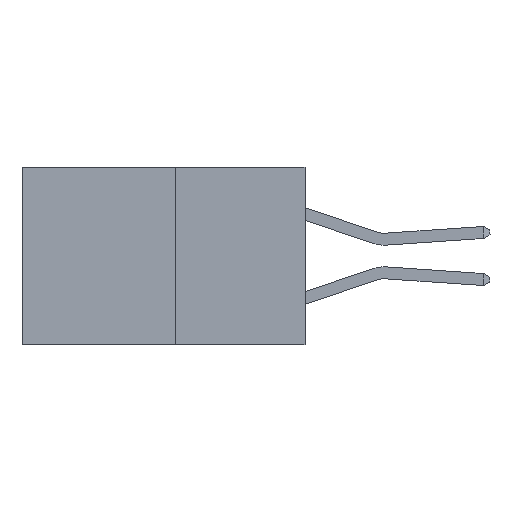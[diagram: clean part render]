
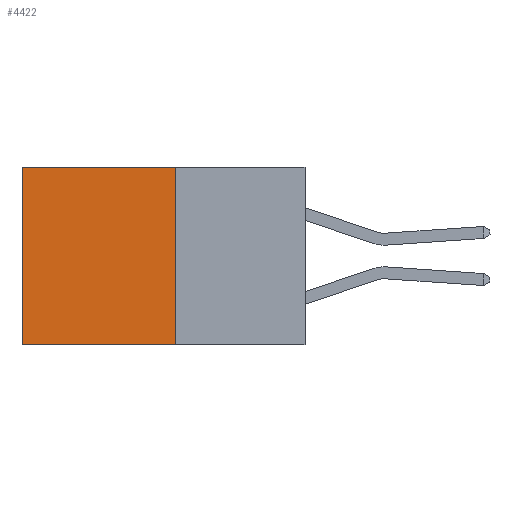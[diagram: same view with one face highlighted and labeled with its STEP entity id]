
A CAD part, left-side view. The second image highlights one B-rep face of the part: STEP entity #4422.
In plain terms, the highlighted planar face has unit normal (-1, 0, 0).
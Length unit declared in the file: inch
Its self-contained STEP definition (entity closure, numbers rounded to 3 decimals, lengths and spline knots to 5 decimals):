
#816 = EDGE_CURVE ( 'NONE', #3870, #5672, #6788, .T. ) ;
#1032 = EDGE_CURVE ( 'NONE', #5672, #4054, #9245, .T. ) ;
#1395 = CARTESIAN_POINT ( 'NONE',  ( 0.277, 0.27, -0.37 ) ) ;
#1865 = CARTESIAN_POINT ( 'NONE',  ( 0.277, 0.59, -0.37 ) ) ;
#2240 = CARTESIAN_POINT ( 'NONE',  ( 0.277, 0.59, 0. ) ) ;
#2380 = CARTESIAN_POINT ( 'NONE',  ( 0.277, 0.27, -0.37 ) ) ;
#2745 = LINE ( 'NONE', #2380, #8759 ) ;
#3063 = EDGE_CURVE ( 'NONE', #7665, #4054, #6095, .T. ) ;
#3579 = CARTESIAN_POINT ( 'NONE',  ( 0.277, 0.59, -0.37 ) ) ;
#3745 = AXIS2_PLACEMENT_3D ( 'NONE', #7727, #7685, #7627 ) ;
#3870 = VERTEX_POINT ( 'NONE', #9996 ) ;
#4031 = FACE_OUTER_BOUND ( 'NONE', #9050, .T. ) ;
#4054 = VERTEX_POINT ( 'NONE', #3579 ) ;
#4422 = ADVANCED_FACE ( 'NONE', ( #4031 ), #7743, .F. ) ;
#4441 = ORIENTED_EDGE ( 'NONE', *, *, #1032, .T. ) ;
#4519 = ORIENTED_EDGE ( 'NONE', *, *, #3063, .F. ) ;
#4556 = ORIENTED_EDGE ( 'NONE', *, *, #5852, .F. ) ;
#4741 = DIRECTION ( 'NONE',  ( 0., 0., -1. ) ) ;
#4990 = CARTESIAN_POINT ( 'NONE',  ( 0.277, 0.27, 0. ) ) ;
#5043 = ORIENTED_EDGE ( 'NONE', *, *, #816, .T. ) ;
#5672 = VERTEX_POINT ( 'NONE', #2240 ) ;
#5852 = EDGE_CURVE ( 'NONE', #3870, #7665, #2745, .T. ) ;
#5855 = VECTOR ( 'NONE', #9581, 39.37008 ) ;
#6095 = LINE ( 'NONE', #1395, #5855 ) ;
#6309 = CARTESIAN_POINT ( 'NONE',  ( 0.277, 0.27, -0.37 ) ) ;
#6533 = VECTOR ( 'NONE', #6803, 39.37008 ) ;
#6788 = LINE ( 'NONE', #4990, #6533 ) ;
#6803 = DIRECTION ( 'NONE',  ( 0., 1., 0. ) ) ;
#7219 = DIRECTION ( 'NONE',  ( 0., 0., -1. ) ) ;
#7627 = DIRECTION ( 'NONE',  ( 0., 0., -1. ) ) ;
#7665 = VERTEX_POINT ( 'NONE', #6309 ) ;
#7685 = DIRECTION ( 'NONE',  ( 1., 0., 0. ) ) ;
#7727 = CARTESIAN_POINT ( 'NONE',  ( 0.277, 0.27, -0.37 ) ) ;
#7743 = PLANE ( 'NONE',  #3745 ) ;
#8759 = VECTOR ( 'NONE', #7219, 39.37008 ) ;
#9027 = VECTOR ( 'NONE', #4741, 39.37008 ) ;
#9050 = EDGE_LOOP ( 'NONE', ( #4441, #4519, #4556, #5043 ) ) ;
#9245 = LINE ( 'NONE', #1865, #9027 ) ;
#9581 = DIRECTION ( 'NONE',  ( 0., 1., 0. ) ) ;
#9996 = CARTESIAN_POINT ( 'NONE',  ( 0.277, 0.27, 0. ) ) ;
